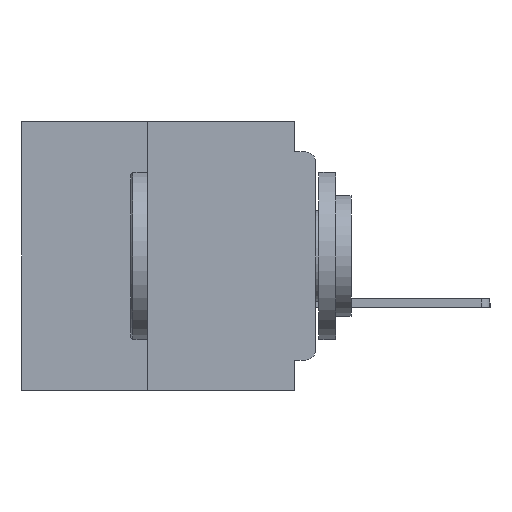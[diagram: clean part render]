
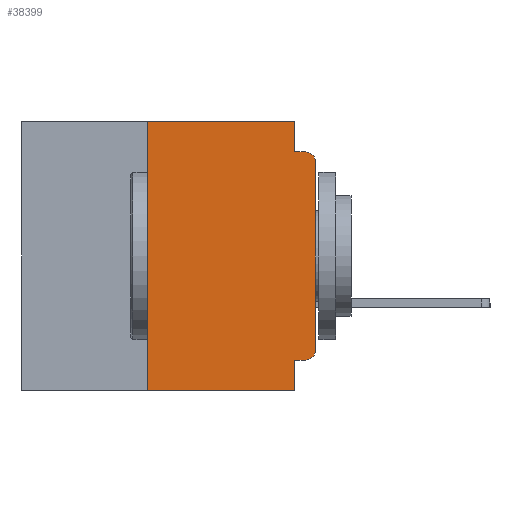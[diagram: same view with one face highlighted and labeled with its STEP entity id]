
A CAD part, left-side view. The second image highlights one B-rep face of the part: STEP entity #38399.
In plain terms, the highlighted planar face has unit normal (-1, 0, 0).
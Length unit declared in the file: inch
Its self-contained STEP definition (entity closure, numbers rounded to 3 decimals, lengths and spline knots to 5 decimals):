
#61 = LINE ( 'NONE', #15624, #32691 ) ;
#255 = CARTESIAN_POINT ( 'NONE',  ( 0., 0.437, 0. ) ) ;
#497 = DIRECTION ( 'NONE',  ( -1., 0., 0. ) ) ;
#2319 = VECTOR ( 'NONE', #10981, 39.37008 ) ;
#2516 = VERTEX_POINT ( 'NONE', #14266 ) ;
#3230 = ORIENTED_EDGE ( 'NONE', *, *, #3650, .F. ) ;
#3298 = VERTEX_POINT ( 'NONE', #26278 ) ;
#3315 = LINE ( 'NONE', #4455, #2319 ) ;
#3606 = EDGE_CURVE ( 'NONE', #3298, #17568, #19811, .T. ) ;
#3650 = EDGE_CURVE ( 'NONE', #18484, #38402, #9124, .T. ) ;
#3787 = ORIENTED_EDGE ( 'NONE', *, *, #15392, .T. ) ;
#4076 = PLANE ( 'NONE',  #41852 ) ;
#4455 = CARTESIAN_POINT ( 'NONE',  ( 0., 0.25, -0.4 ) ) ;
#5802 = EDGE_CURVE ( 'NONE', #3298, #37220, #3315, .T. ) ;
#7090 = DIRECTION ( 'NONE',  ( 0., 0., -1. ) ) ;
#7329 = CARTESIAN_POINT ( 'NONE',  ( 0., 0.437, 0. ) ) ;
#7634 = EDGE_LOOP ( 'NONE', ( #41598, #15784, #3230, #38710, #19665, #28090, #33608, #9535, #14281, #3787 ) ) ;
#7976 = EDGE_CURVE ( 'NONE', #20723, #18484, #28842, .T. ) ;
#9124 = LINE ( 'NONE', #17585, #34162 ) ;
#9197 = DIRECTION ( 'NONE',  ( 0., 0., 1. ) ) ;
#9535 = ORIENTED_EDGE ( 'NONE', *, *, #39398, .F. ) ;
#10597 = DIRECTION ( 'NONE',  ( 1., 0., 0. ) ) ;
#10981 = DIRECTION ( 'NONE',  ( 0., 0., 1. ) ) ;
#11157 = VECTOR ( 'NONE', #19038, 39.37008 ) ;
#11459 = DIRECTION ( 'NONE',  ( 0., 1., 0. ) ) ;
#11495 = CARTESIAN_POINT ( 'NONE',  ( 0., 0.015, -0.355 ) ) ;
#11996 = CARTESIAN_POINT ( 'NONE',  ( 0., 0.015, -0.34 ) ) ;
#13555 = CARTESIAN_POINT ( 'NONE',  ( 0., 0.25, 0. ) ) ;
#13886 = CARTESIAN_POINT ( 'NONE',  ( 0., 0.031, -0.355 ) ) ;
#14266 = CARTESIAN_POINT ( 'NONE',  ( 0., 0., -0.34 ) ) ;
#14281 = ORIENTED_EDGE ( 'NONE', *, *, #30731, .F. ) ;
#15298 = DIRECTION ( 'NONE',  ( 0., 0., -1. ) ) ;
#15392 = EDGE_CURVE ( 'NONE', #16211, #2516, #28225, .T. ) ;
#15624 = CARTESIAN_POINT ( 'NONE',  ( 0., 0., 0. ) ) ;
#15784 = ORIENTED_EDGE ( 'NONE', *, *, #19730, .T. ) ;
#16211 = VERTEX_POINT ( 'NONE', #11495 ) ;
#17568 = VERTEX_POINT ( 'NONE', #38932 ) ;
#17585 = CARTESIAN_POINT ( 'NONE',  ( 0., 0., -0.045 ) ) ;
#17648 = DIRECTION ( 'NONE',  ( 0., -1., 0. ) ) ;
#17855 = CARTESIAN_POINT ( 'NONE',  ( 0., 0.031, 0. ) ) ;
#17862 = CARTESIAN_POINT ( 'NONE',  ( 0., 0., -0.355 ) ) ;
#18418 = AXIS2_PLACEMENT_3D ( 'NONE', #19940, #497, #23252 ) ;
#18484 = VERTEX_POINT ( 'NONE', #27187 ) ;
#18926 = EDGE_CURVE ( 'NONE', #2516, #41660, #61, .T. ) ;
#19038 = DIRECTION ( 'NONE',  ( 0., -1., 0. ) ) ;
#19312 = CARTESIAN_POINT ( 'NONE',  ( 0., 0.437, -0.4 ) ) ;
#19665 = ORIENTED_EDGE ( 'NONE', *, *, #36499, .F. ) ;
#19730 = EDGE_CURVE ( 'NONE', #41660, #38402, #35675, .T. ) ;
#19811 = LINE ( 'NONE', #19312, #11157 ) ;
#19940 = CARTESIAN_POINT ( 'NONE',  ( 0., 0.015, -0.06 ) ) ;
#20723 = VERTEX_POINT ( 'NONE', #28790 ) ;
#21146 = DIRECTION ( 'NONE',  ( 0., 0., -1. ) ) ;
#22121 = AXIS2_PLACEMENT_3D ( 'NONE', #11996, #34854, #15298 ) ;
#23252 = DIRECTION ( 'NONE',  ( 0., 0., -1. ) ) ;
#23582 = CARTESIAN_POINT ( 'NONE',  ( 0., 0.015, -0.045 ) ) ;
#26278 = CARTESIAN_POINT ( 'NONE',  ( 0., 0.25, -0.4 ) ) ;
#26305 = DIRECTION ( 'NONE',  ( 0., -1., 0. ) ) ;
#26336 = VERTEX_POINT ( 'NONE', #13886 ) ;
#26639 = CARTESIAN_POINT ( 'NONE',  ( 0., 0.031, -0.4 ) ) ;
#27187 = CARTESIAN_POINT ( 'NONE',  ( 0., 0.031, -0.045 ) ) ;
#28090 = ORIENTED_EDGE ( 'NONE', *, *, #5802, .F. ) ;
#28225 = CIRCLE ( 'NONE', #22121, 0.015 ) ;
#28790 = CARTESIAN_POINT ( 'NONE',  ( 0., 0.031, 0. ) ) ;
#28842 = LINE ( 'NONE', #17855, #29847 ) ;
#29332 = LINE ( 'NONE', #26639, #36972 ) ;
#29527 = LINE ( 'NONE', #255, #39183 ) ;
#29847 = VECTOR ( 'NONE', #21146, 39.37008 ) ;
#30731 = EDGE_CURVE ( 'NONE', #16211, #26336, #35443, .T. ) ;
#32691 = VECTOR ( 'NONE', #9197, 39.37008 ) ;
#33455 = DIRECTION ( 'NONE',  ( 0., 0., -1. ) ) ;
#33608 = ORIENTED_EDGE ( 'NONE', *, *, #3606, .T. ) ;
#34162 = VECTOR ( 'NONE', #17648, 39.37008 ) ;
#34854 = DIRECTION ( 'NONE',  ( -1., 0., 0. ) ) ;
#35398 = CARTESIAN_POINT ( 'NONE',  ( 0., 0., -0.06 ) ) ;
#35443 = LINE ( 'NONE', #17862, #42002 ) ;
#35675 = CIRCLE ( 'NONE', #18418, 0.015 ) ;
#36499 = EDGE_CURVE ( 'NONE', #37220, #20723, #29527, .T. ) ;
#36972 = VECTOR ( 'NONE', #7090, 39.37008 ) ;
#37220 = VERTEX_POINT ( 'NONE', #13555 ) ;
#38399 = ADVANCED_FACE ( 'NONE', ( #41526 ), #4076, .F. ) ;
#38402 = VERTEX_POINT ( 'NONE', #23582 ) ;
#38710 = ORIENTED_EDGE ( 'NONE', *, *, #7976, .F. ) ;
#38932 = CARTESIAN_POINT ( 'NONE',  ( 0., 0.031, -0.4 ) ) ;
#39183 = VECTOR ( 'NONE', #26305, 39.37008 ) ;
#39398 = EDGE_CURVE ( 'NONE', #26336, #17568, #29332, .T. ) ;
#41526 = FACE_OUTER_BOUND ( 'NONE', #7634, .T. ) ;
#41598 = ORIENTED_EDGE ( 'NONE', *, *, #18926, .T. ) ;
#41660 = VERTEX_POINT ( 'NONE', #35398 ) ;
#41852 = AXIS2_PLACEMENT_3D ( 'NONE', #7329, #10597, #33455 ) ;
#42002 = VECTOR ( 'NONE', #11459, 39.37008 ) ;
